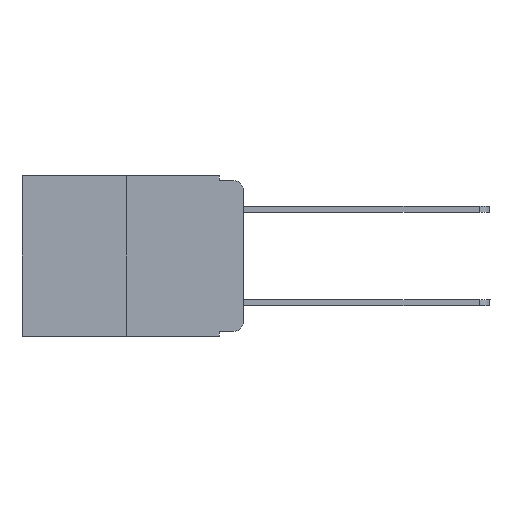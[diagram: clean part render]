
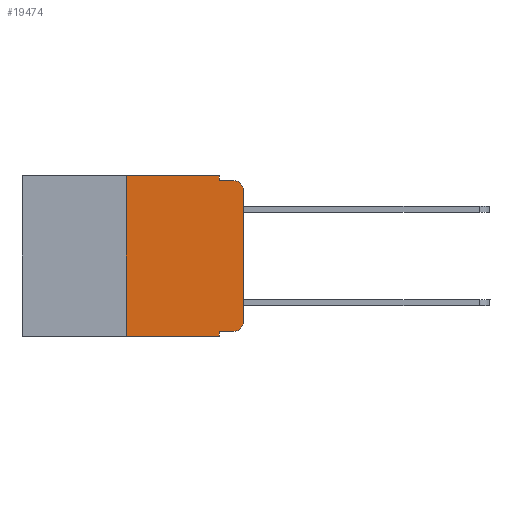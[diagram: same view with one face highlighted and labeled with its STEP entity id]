
A CAD part, left-side view. The second image highlights one B-rep face of the part: STEP entity #19474.
In plain terms, the highlighted planar face has unit normal (-1, 0, 0).
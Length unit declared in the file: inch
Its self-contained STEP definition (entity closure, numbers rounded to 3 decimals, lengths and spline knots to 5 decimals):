
#35 = ORIENTED_EDGE ( 'NONE', *, *, #3563, .F. ) ;
#126 = LINE ( 'NONE', #15087, #10273 ) ;
#245 = CARTESIAN_POINT ( 'NONE',  ( 0., 0.02, -0.313 ) ) ;
#735 = VERTEX_POINT ( 'NONE', #16667 ) ;
#1138 = VERTEX_POINT ( 'NONE', #12233 ) ;
#1181 = ORIENTED_EDGE ( 'NONE', *, *, #8387, .F. ) ;
#1311 = CARTESIAN_POINT ( 'NONE',  ( 0., 0.051, 0. ) ) ;
#1547 = ORIENTED_EDGE ( 'NONE', *, *, #9217, .T. ) ;
#1672 = EDGE_CURVE ( 'NONE', #12827, #15334, #16588, .T. ) ;
#2060 = CIRCLE ( 'NONE', #13190, 0.02 ) ;
#2296 = LINE ( 'NONE', #17433, #19346 ) ;
#2316 = DIRECTION ( 'NONE',  ( 0., 0., -1. ) ) ;
#2558 = DIRECTION ( 'NONE',  ( 1., 0., 0. ) ) ;
#2774 = LINE ( 'NONE', #8833, #13014 ) ;
#3259 = CARTESIAN_POINT ( 'NONE',  ( 0., 0.473, 0. ) ) ;
#3563 = EDGE_CURVE ( 'NONE', #8866, #12827, #126, .T. ) ;
#3716 = CARTESIAN_POINT ( 'NONE',  ( 0., 0.02, -0.03 ) ) ;
#3795 = DIRECTION ( 'NONE',  ( 0., 0., -1. ) ) ;
#4149 = FACE_OUTER_BOUND ( 'NONE', #17252, .T. ) ;
#4524 = DIRECTION ( 'NONE',  ( 0., 0., 1. ) ) ;
#4955 = ORIENTED_EDGE ( 'NONE', *, *, #7776, .F. ) ;
#5247 = VERTEX_POINT ( 'NONE', #12002 ) ;
#5590 = LINE ( 'NONE', #19649, #10292 ) ;
#5643 = LINE ( 'NONE', #19602, #10853 ) ;
#5848 = CARTESIAN_POINT ( 'NONE',  ( 0., 0.051, -0.01 ) ) ;
#6124 = EDGE_CURVE ( 'NONE', #1138, #6613, #2060, .T. ) ;
#6335 = DIRECTION ( 'NONE',  ( -1., 0., 0. ) ) ;
#6613 = VERTEX_POINT ( 'NONE', #9848 ) ;
#6987 = ORIENTED_EDGE ( 'NONE', *, *, #18818, .T. ) ;
#7370 = DIRECTION ( 'NONE',  ( 0., 0., -1. ) ) ;
#7411 = ORIENTED_EDGE ( 'NONE', *, *, #1672, .F. ) ;
#7776 = EDGE_CURVE ( 'NONE', #10319, #735, #2296, .T. ) ;
#8241 = CARTESIAN_POINT ( 'NONE',  ( 0., 0.473, -0.343 ) ) ;
#8316 = AXIS2_PLACEMENT_3D ( 'NONE', #245, #6335, #9804 ) ;
#8338 = LINE ( 'NONE', #8241, #19418 ) ;
#8387 = EDGE_CURVE ( 'NONE', #8413, #6613, #5643, .T. ) ;
#8413 = VERTEX_POINT ( 'NONE', #5848 ) ;
#8535 = EDGE_CURVE ( 'NONE', #5247, #11362, #13100, .T. ) ;
#8833 = CARTESIAN_POINT ( 'NONE',  ( 0., 0., 0. ) ) ;
#8866 = VERTEX_POINT ( 'NONE', #16862 ) ;
#9173 = EDGE_CURVE ( 'NONE', #15334, #8413, #19262, .T. ) ;
#9217 = EDGE_CURVE ( 'NONE', #10319, #5247, #5590, .T. ) ;
#9804 = DIRECTION ( 'NONE',  ( 0., 0., -1. ) ) ;
#9848 = CARTESIAN_POINT ( 'NONE',  ( 0., 0.02, -0.01 ) ) ;
#9913 = DIRECTION ( 'NONE',  ( 0., 0., -1. ) ) ;
#10032 = DIRECTION ( 'NONE',  ( 0., -1., 0. ) ) ;
#10273 = VECTOR ( 'NONE', #4524, 39.37008 ) ;
#10292 = VECTOR ( 'NONE', #10571, 39.37008 ) ;
#10319 = VERTEX_POINT ( 'NONE', #11179 ) ;
#10571 = DIRECTION ( 'NONE',  ( 0., -1., 0. ) ) ;
#10853 = VECTOR ( 'NONE', #10032, 39.37008 ) ;
#10910 = DIRECTION ( 'NONE',  ( 0., -1., 0. ) ) ;
#11179 = CARTESIAN_POINT ( 'NONE',  ( 0., 0.051, -0.333 ) ) ;
#11293 = ORIENTED_EDGE ( 'NONE', *, *, #6124, .T. ) ;
#11362 = VERTEX_POINT ( 'NONE', #18712 ) ;
#11481 = VECTOR ( 'NONE', #10910, 39.37008 ) ;
#12002 = CARTESIAN_POINT ( 'NONE',  ( 0., 0.02, -0.333 ) ) ;
#12233 = CARTESIAN_POINT ( 'NONE',  ( 0., 0., -0.03 ) ) ;
#12734 = DIRECTION ( 'NONE',  ( 0., -1., 0. ) ) ;
#12739 = AXIS2_PLACEMENT_3D ( 'NONE', #16198, #2558, #9913 ) ;
#12827 = VERTEX_POINT ( 'NONE', #16600 ) ;
#13014 = VECTOR ( 'NONE', #14910, 39.37008 ) ;
#13100 = CIRCLE ( 'NONE', #8316, 0.02 ) ;
#13190 = AXIS2_PLACEMENT_3D ( 'NONE', #3716, #17455, #2316 ) ;
#14321 = ORIENTED_EDGE ( 'NONE', *, *, #8535, .T. ) ;
#14910 = DIRECTION ( 'NONE',  ( 0., 0., 1. ) ) ;
#15087 = CARTESIAN_POINT ( 'NONE',  ( 0., 0.25, 0. ) ) ;
#15091 = CARTESIAN_POINT ( 'NONE',  ( 0., 0.051, 0. ) ) ;
#15334 = VERTEX_POINT ( 'NONE', #15091 ) ;
#16198 = CARTESIAN_POINT ( 'NONE',  ( 0., 0.473, 0. ) ) ;
#16588 = LINE ( 'NONE', #3259, #11481 ) ;
#16600 = CARTESIAN_POINT ( 'NONE',  ( 0., 0.25, 0. ) ) ;
#16667 = CARTESIAN_POINT ( 'NONE',  ( 0., 0.051, -0.343 ) ) ;
#16862 = CARTESIAN_POINT ( 'NONE',  ( 0., 0.25, -0.343 ) ) ;
#17252 = EDGE_LOOP ( 'NONE', ( #17477, #11293, #1181, #18914, #7411, #35, #6987, #4955, #1547, #14321 ) ) ;
#17291 = VECTOR ( 'NONE', #7370, 39.37008 ) ;
#17433 = CARTESIAN_POINT ( 'NONE',  ( 0., 0.051, 0. ) ) ;
#17455 = DIRECTION ( 'NONE',  ( -1., 0., 0. ) ) ;
#17477 = ORIENTED_EDGE ( 'NONE', *, *, #17897, .T. ) ;
#17897 = EDGE_CURVE ( 'NONE', #11362, #1138, #2774, .T. ) ;
#18712 = CARTESIAN_POINT ( 'NONE',  ( 0., 0., -0.313 ) ) ;
#18818 = EDGE_CURVE ( 'NONE', #8866, #735, #8338, .T. ) ;
#18914 = ORIENTED_EDGE ( 'NONE', *, *, #9173, .F. ) ;
#19262 = LINE ( 'NONE', #1311, #17291 ) ;
#19346 = VECTOR ( 'NONE', #3795, 39.37008 ) ;
#19418 = VECTOR ( 'NONE', #12734, 39.37008 ) ;
#19474 = ADVANCED_FACE ( 'NONE', ( #4149 ), #19494, .F. ) ;
#19494 = PLANE ( 'NONE',  #12739 ) ;
#19602 = CARTESIAN_POINT ( 'NONE',  ( 0., 0.051, -0.01 ) ) ;
#19649 = CARTESIAN_POINT ( 'NONE',  ( 0., 0.051, -0.333 ) ) ;
